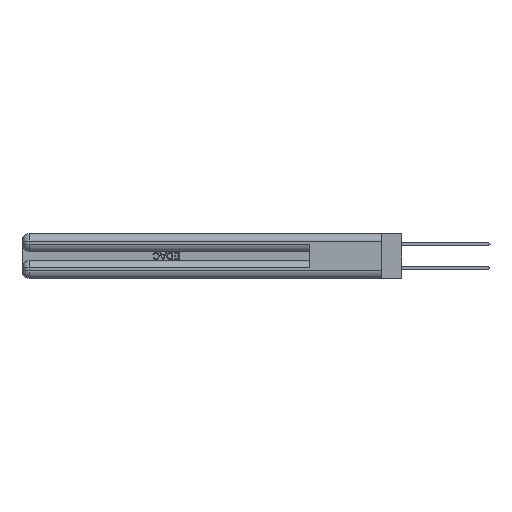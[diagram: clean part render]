
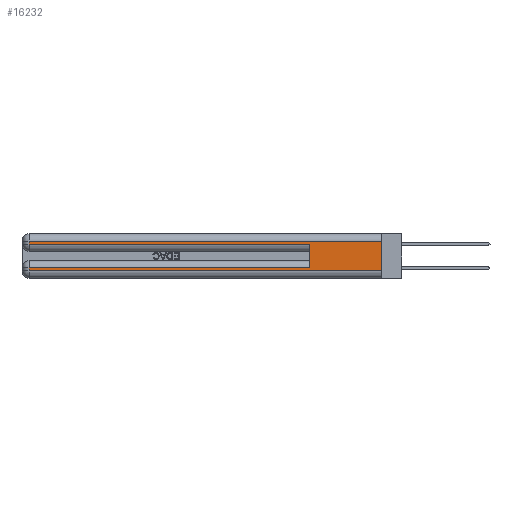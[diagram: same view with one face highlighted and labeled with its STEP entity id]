
A CAD part, left-side view. The second image highlights one B-rep face of the part: STEP entity #16232.
In plain terms, the highlighted planar face has unit normal (-1, 0, 0).
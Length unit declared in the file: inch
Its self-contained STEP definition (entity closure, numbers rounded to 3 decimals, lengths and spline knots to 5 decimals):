
#730 = EDGE_CURVE ( 'NONE', #46172, #1544, #12533, .T. ) ;
#1544 = VERTEX_POINT ( 'NONE', #38319 ) ;
#1562 = EDGE_CURVE ( 'NONE', #45190, #23079, #44797, .T. ) ;
#1658 = CARTESIAN_POINT ( 'NONE',  ( 0., 2.94, 0.285 ) ) ;
#1789 = VECTOR ( 'NONE', #40454, 39.37008 ) ;
#2640 = ORIENTED_EDGE ( 'NONE', *, *, #730, .T. ) ;
#2719 = VECTOR ( 'NONE', #30649, 39.37008 ) ;
#5220 = EDGE_CURVE ( 'NONE', #23079, #22764, #26346, .T. ) ;
#5661 = FACE_OUTER_BOUND ( 'NONE', #16025, .T. ) ;
#7269 = ORIENTED_EDGE ( 'NONE', *, *, #29589, .F. ) ;
#7304 = VECTOR ( 'NONE', #38468, 39.37008 ) ;
#7588 = DIRECTION ( 'NONE',  ( 0., 0., -1. ) ) ;
#8424 = DIRECTION ( 'NONE',  ( 0., 0., 1. ) ) ;
#9684 = CARTESIAN_POINT ( 'NONE',  ( 0., 0.6, 0.085 ) ) ;
#10705 = CARTESIAN_POINT ( 'NONE',  ( 0., 2.94, 0.31 ) ) ;
#11356 = CARTESIAN_POINT ( 'NONE',  ( 0., 0., 0.31 ) ) ;
#11429 = CARTESIAN_POINT ( 'NONE',  ( 0., 0., 0.06 ) ) ;
#11870 = ORIENTED_EDGE ( 'NONE', *, *, #5220, .T. ) ;
#12533 = LINE ( 'NONE', #22645, #2719 ) ;
#12868 = LINE ( 'NONE', #40435, #23667 ) ;
#13785 = DIRECTION ( 'NONE',  ( 0., 0., -1. ) ) ;
#15287 = ORIENTED_EDGE ( 'NONE', *, *, #44584, .T. ) ;
#15759 = CARTESIAN_POINT ( 'NONE',  ( 0., 0.6, 0.145 ) ) ;
#16025 = EDGE_LOOP ( 'NONE', ( #7269, #36322, #11870, #15287, #28386, #2640, #22120, #43667 ) ) ;
#16232 = ADVANCED_FACE ( 'NONE', ( #5661 ), #22081, .F. ) ;
#16710 = CARTESIAN_POINT ( 'NONE',  ( 0., 0., 0.31 ) ) ;
#17591 = CARTESIAN_POINT ( 'NONE',  ( 0., 0., 0.285 ) ) ;
#18704 = DIRECTION ( 'NONE',  ( 0., 0., -1. ) ) ;
#20859 = EDGE_CURVE ( 'NONE', #1544, #35518, #12868, .T. ) ;
#21301 = LINE ( 'NONE', #36868, #1789 ) ;
#21710 = LINE ( 'NONE', #17591, #22837 ) ;
#21954 = EDGE_CURVE ( 'NONE', #46172, #40443, #34979, .T. ) ;
#22081 = PLANE ( 'NONE',  #38303 ) ;
#22120 = ORIENTED_EDGE ( 'NONE', *, *, #20859, .T. ) ;
#22645 = CARTESIAN_POINT ( 'NONE',  ( 0., 0., 0.085 ) ) ;
#22649 = VECTOR ( 'NONE', #29509, 39.37008 ) ;
#22764 = VERTEX_POINT ( 'NONE', #1658 ) ;
#22837 = VECTOR ( 'NONE', #42984, 39.37008 ) ;
#23079 = VERTEX_POINT ( 'NONE', #10705 ) ;
#23667 = VECTOR ( 'NONE', #18704, 39.37008 ) ;
#25718 = CARTESIAN_POINT ( 'NONE',  ( 0., 0., 0.37 ) ) ;
#25810 = CARTESIAN_POINT ( 'NONE',  ( 0., 0., 0.37 ) ) ;
#26346 = LINE ( 'NONE', #31957, #34921 ) ;
#28386 = ORIENTED_EDGE ( 'NONE', *, *, #21954, .F. ) ;
#29411 = DIRECTION ( 'NONE',  ( 1., 0., 0. ) ) ;
#29509 = DIRECTION ( 'NONE',  ( 0., 0., -1. ) ) ;
#29589 = EDGE_CURVE ( 'NONE', #45190, #42534, #38549, .T. ) ;
#30649 = DIRECTION ( 'NONE',  ( 0., 1., 0. ) ) ;
#31957 = CARTESIAN_POINT ( 'NONE',  ( 0., 2.94, 0.37 ) ) ;
#34640 = CARTESIAN_POINT ( 'NONE',  ( 0., 0.6, 0.285 ) ) ;
#34921 = VECTOR ( 'NONE', #13785, 39.37008 ) ;
#34979 = LINE ( 'NONE', #15759, #45667 ) ;
#35518 = VERTEX_POINT ( 'NONE', #38226 ) ;
#36322 = ORIENTED_EDGE ( 'NONE', *, *, #1562, .T. ) ;
#36868 = CARTESIAN_POINT ( 'NONE',  ( 0., 0., 0.06 ) ) ;
#38226 = CARTESIAN_POINT ( 'NONE',  ( 0., 2.94, 0.06 ) ) ;
#38303 = AXIS2_PLACEMENT_3D ( 'NONE', #25718, #29411, #7588 ) ;
#38319 = CARTESIAN_POINT ( 'NONE',  ( 0., 2.94, 0.085 ) ) ;
#38468 = DIRECTION ( 'NONE',  ( 0., 1., 0. ) ) ;
#38549 = LINE ( 'NONE', #25810, #22649 ) ;
#40435 = CARTESIAN_POINT ( 'NONE',  ( 0., 2.94, 0.37 ) ) ;
#40443 = VERTEX_POINT ( 'NONE', #34640 ) ;
#40454 = DIRECTION ( 'NONE',  ( 0., -1., 0. ) ) ;
#42508 = EDGE_CURVE ( 'NONE', #35518, #42534, #21301, .T. ) ;
#42534 = VERTEX_POINT ( 'NONE', #11429 ) ;
#42984 = DIRECTION ( 'NONE',  ( 0., -1., 0. ) ) ;
#43667 = ORIENTED_EDGE ( 'NONE', *, *, #42508, .T. ) ;
#44584 = EDGE_CURVE ( 'NONE', #22764, #40443, #21710, .T. ) ;
#44797 = LINE ( 'NONE', #16710, #7304 ) ;
#45190 = VERTEX_POINT ( 'NONE', #11356 ) ;
#45667 = VECTOR ( 'NONE', #8424, 39.37008 ) ;
#46172 = VERTEX_POINT ( 'NONE', #9684 ) ;
